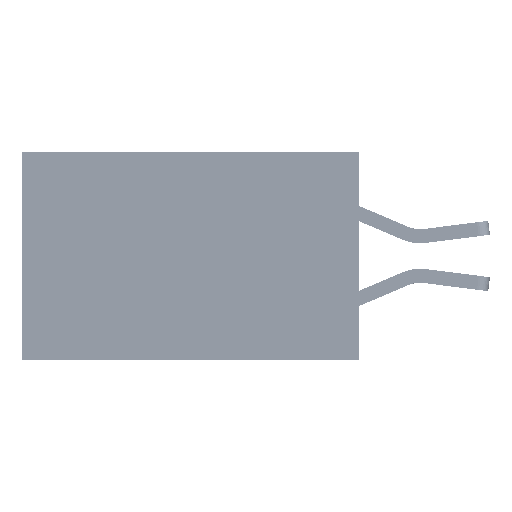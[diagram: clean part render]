
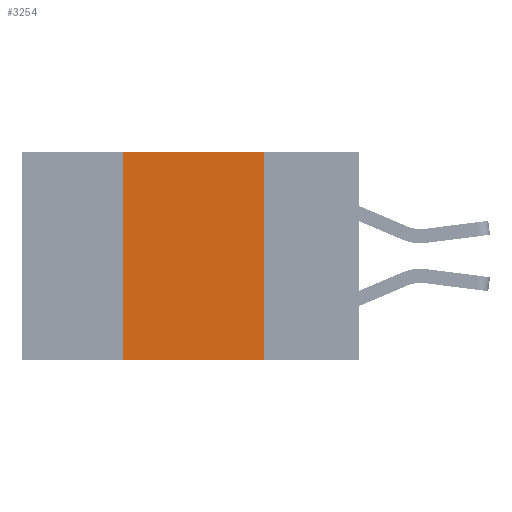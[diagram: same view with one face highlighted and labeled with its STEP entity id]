
A CAD part, left-side view. The second image highlights one B-rep face of the part: STEP entity #3254.
In plain terms, the highlighted planar face has unit normal (-1, 0, 0).
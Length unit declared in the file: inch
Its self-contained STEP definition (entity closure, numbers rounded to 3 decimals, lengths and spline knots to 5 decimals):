
#106 = LINE ( 'NONE', #28429, #37808 ) ;
#1592 = VERTEX_POINT ( 'NONE', #3269 ) ;
#3254 = ADVANCED_FACE ( 'NONE', ( #29539 ), #17755, .F. ) ;
#3269 = CARTESIAN_POINT ( 'NONE',  ( 0., 0.17, -0.37 ) ) ;
#5799 = DIRECTION ( 'NONE',  ( 1., 0., 0. ) ) ;
#7027 = ORIENTED_EDGE ( 'NONE', *, *, #18421, .F. ) ;
#8164 = EDGE_LOOP ( 'NONE', ( #20088, #22008, #7027, #27064 ) ) ;
#10799 = DIRECTION ( 'NONE',  ( 0., -1., 0. ) ) ;
#10814 = VECTOR ( 'NONE', #19924, 39.37008 ) ;
#12887 = CARTESIAN_POINT ( 'NONE',  ( 0., 0.42, 0. ) ) ;
#14088 = LINE ( 'NONE', #37153, #37275 ) ;
#14208 = CARTESIAN_POINT ( 'NONE',  ( 0., 0.6, 0. ) ) ;
#14775 = VECTOR ( 'NONE', #38343, 39.37008 ) ;
#15272 = EDGE_CURVE ( 'NONE', #28741, #21002, #106, .T. ) ;
#16539 = CARTESIAN_POINT ( 'NONE',  ( 0., 0.6, -0.37 ) ) ;
#17399 = CARTESIAN_POINT ( 'NONE',  ( 0., 0.17, 0. ) ) ;
#17755 = PLANE ( 'NONE',  #27562 ) ;
#18421 = EDGE_CURVE ( 'NONE', #21550, #28741, #32400, .T. ) ;
#19924 = DIRECTION ( 'NONE',  ( 0., -1., 0. ) ) ;
#20088 = ORIENTED_EDGE ( 'NONE', *, *, #38467, .F. ) ;
#21002 = VERTEX_POINT ( 'NONE', #17399 ) ;
#21337 = EDGE_CURVE ( 'NONE', #21550, #1592, #26577, .T. ) ;
#21550 = VERTEX_POINT ( 'NONE', #29719 ) ;
#22008 = ORIENTED_EDGE ( 'NONE', *, *, #15272, .F. ) ;
#23369 = CARTESIAN_POINT ( 'NONE',  ( 0., 0.42, 0. ) ) ;
#26577 = LINE ( 'NONE', #16539, #10814 ) ;
#27064 = ORIENTED_EDGE ( 'NONE', *, *, #21337, .T. ) ;
#27562 = AXIS2_PLACEMENT_3D ( 'NONE', #14208, #5799, #32418 ) ;
#28429 = CARTESIAN_POINT ( 'NONE',  ( 0., 0.6, 0. ) ) ;
#28741 = VERTEX_POINT ( 'NONE', #12887 ) ;
#29539 = FACE_OUTER_BOUND ( 'NONE', #8164, .T. ) ;
#29719 = CARTESIAN_POINT ( 'NONE',  ( 0., 0.42, -0.37 ) ) ;
#31584 = DIRECTION ( 'NONE',  ( 0., 0., -1. ) ) ;
#32400 = LINE ( 'NONE', #23369, #14775 ) ;
#32418 = DIRECTION ( 'NONE',  ( 0., 0., -1. ) ) ;
#37153 = CARTESIAN_POINT ( 'NONE',  ( 0., 0.17, 0. ) ) ;
#37275 = VECTOR ( 'NONE', #31584, 39.37008 ) ;
#37808 = VECTOR ( 'NONE', #10799, 39.37008 ) ;
#38343 = DIRECTION ( 'NONE',  ( 0., 0., 1. ) ) ;
#38467 = EDGE_CURVE ( 'NONE', #21002, #1592, #14088, .T. ) ;
